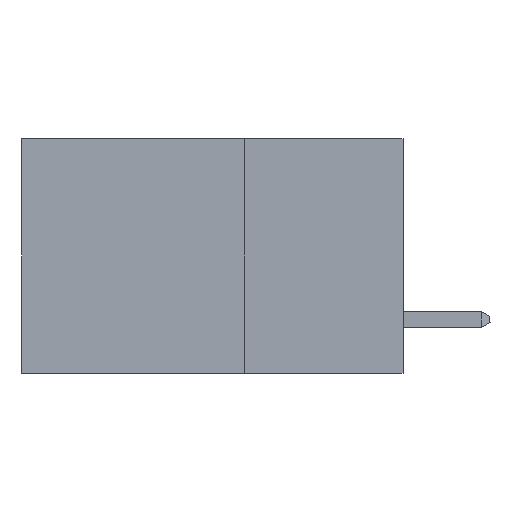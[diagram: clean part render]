
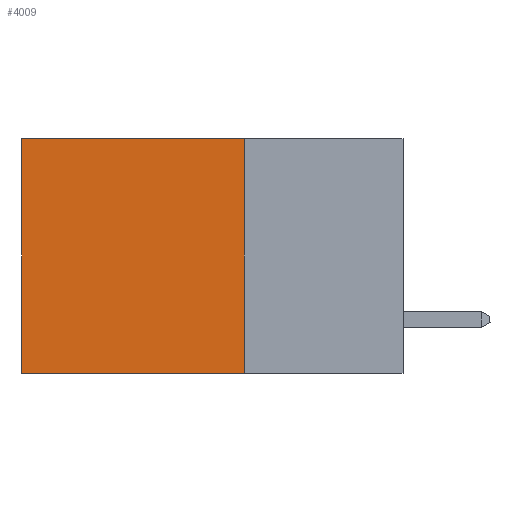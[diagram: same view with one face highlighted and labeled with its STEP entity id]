
A CAD part, left-side view. The second image highlights one B-rep face of the part: STEP entity #4009.
In plain terms, the highlighted planar face has unit normal (-1, 0, 0).
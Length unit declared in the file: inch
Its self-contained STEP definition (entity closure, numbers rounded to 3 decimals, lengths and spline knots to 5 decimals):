
#573 = ORIENTED_EDGE ( 'NONE', *, *, #12231, .T. ) ;
#636 = EDGE_LOOP ( 'NONE', ( #573, #11862, #9889, #7249 ) ) ;
#833 = VERTEX_POINT ( 'NONE', #7052 ) ;
#918 = LINE ( 'NONE', #11345, #2811 ) ;
#1067 = EDGE_CURVE ( 'NONE', #2606, #833, #7797, .T. ) ;
#1358 = DIRECTION ( 'NONE',  ( 0., 0., -1. ) ) ;
#2606 = VERTEX_POINT ( 'NONE', #2839 ) ;
#2811 = VECTOR ( 'NONE', #12649, 39.37008 ) ;
#2839 = CARTESIAN_POINT ( 'NONE',  ( 0.2875, 0.25, 0. ) ) ;
#3776 = VECTOR ( 'NONE', #4304, 39.37008 ) ;
#3782 = EDGE_CURVE ( 'NONE', #833, #8060, #5642, .T. ) ;
#4009 = ADVANCED_FACE ( 'NONE', ( #6713 ), #7402, .F. ) ;
#4036 = CARTESIAN_POINT ( 'NONE',  ( 0.2875, 0.6, 0. ) ) ;
#4115 = VERTEX_POINT ( 'NONE', #4036 ) ;
#4304 = DIRECTION ( 'NONE',  ( 0., 1., 0. ) ) ;
#4330 = VECTOR ( 'NONE', #12207, 39.37008 ) ;
#4728 = CARTESIAN_POINT ( 'NONE',  ( 0.2875, 0.6, -0.37 ) ) ;
#5278 = CARTESIAN_POINT ( 'NONE',  ( 0.2875, 0.25, 0. ) ) ;
#5642 = LINE ( 'NONE', #9233, #3776 ) ;
#6000 = CARTESIAN_POINT ( 'NONE',  ( 0.2875, 0.25, 0. ) ) ;
#6713 = FACE_OUTER_BOUND ( 'NONE', #636, .T. ) ;
#6996 = DIRECTION ( 'NONE',  ( 0., 0., -1. ) ) ;
#7052 = CARTESIAN_POINT ( 'NONE',  ( 0.2875, 0.25, -0.37 ) ) ;
#7249 = ORIENTED_EDGE ( 'NONE', *, *, #11227, .T. ) ;
#7402 = PLANE ( 'NONE',  #10093 ) ;
#7797 = LINE ( 'NONE', #6000, #10175 ) ;
#8060 = VERTEX_POINT ( 'NONE', #4728 ) ;
#8720 = LINE ( 'NONE', #10204, #4330 ) ;
#9233 = CARTESIAN_POINT ( 'NONE',  ( 0.2875, 0.25, -0.37 ) ) ;
#9889 = ORIENTED_EDGE ( 'NONE', *, *, #1067, .F. ) ;
#10093 = AXIS2_PLACEMENT_3D ( 'NONE', #5278, #10350, #1358 ) ;
#10175 = VECTOR ( 'NONE', #6996, 39.37008 ) ;
#10204 = CARTESIAN_POINT ( 'NONE',  ( 0.2875, 0.6, 0. ) ) ;
#10350 = DIRECTION ( 'NONE',  ( 1., 0., 0. ) ) ;
#11227 = EDGE_CURVE ( 'NONE', #2606, #4115, #918, .T. ) ;
#11345 = CARTESIAN_POINT ( 'NONE',  ( 0.2875, 0.25, 0. ) ) ;
#11862 = ORIENTED_EDGE ( 'NONE', *, *, #3782, .F. ) ;
#12207 = DIRECTION ( 'NONE',  ( 0., 0., -1. ) ) ;
#12231 = EDGE_CURVE ( 'NONE', #4115, #8060, #8720, .T. ) ;
#12649 = DIRECTION ( 'NONE',  ( 0., 1., 0. ) ) ;
